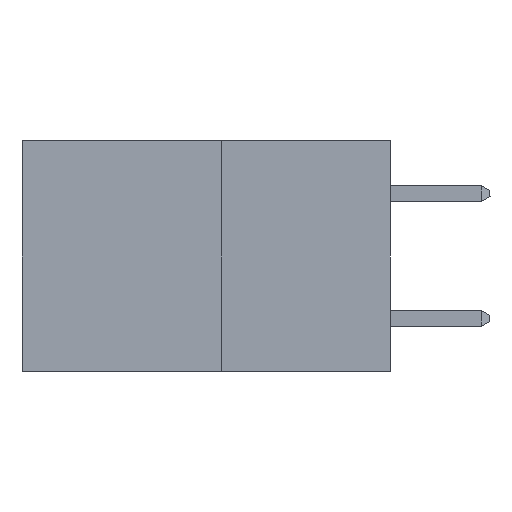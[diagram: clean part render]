
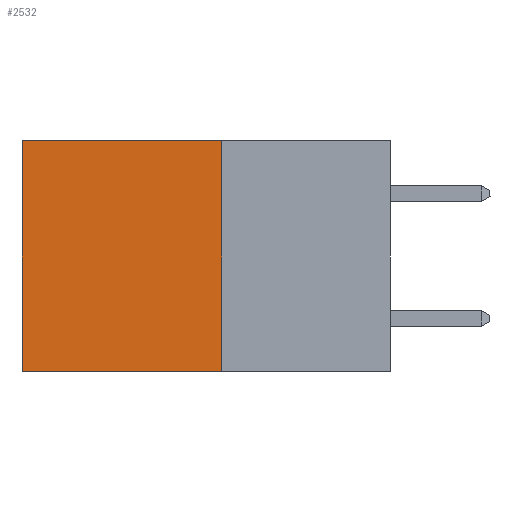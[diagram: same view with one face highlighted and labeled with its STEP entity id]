
A CAD part, left-side view. The second image highlights one B-rep face of the part: STEP entity #2532.
In plain terms, the highlighted planar face has unit normal (-1, 0, 0).
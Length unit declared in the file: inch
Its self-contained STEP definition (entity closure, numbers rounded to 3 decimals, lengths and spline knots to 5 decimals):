
#1038 = LINE ( 'NONE', #13134, #4888 ) ;
#1607 = LINE ( 'NONE', #19316, #9572 ) ;
#2513 = EDGE_CURVE ( 'NONE', #14275, #5086, #7500, .T. ) ;
#2532 = ADVANCED_FACE ( 'NONE', ( #10692 ), #6028, .F. ) ;
#2964 = VERTEX_POINT ( 'NONE', #14074 ) ;
#3160 = ORIENTED_EDGE ( 'NONE', *, *, #2513, .F. ) ;
#3594 = EDGE_LOOP ( 'NONE', ( #10285, #3160, #4442, #5634 ) ) ;
#3852 = VERTEX_POINT ( 'NONE', #9405 ) ;
#4442 = ORIENTED_EDGE ( 'NONE', *, *, #13285, .F. ) ;
#4865 = CARTESIAN_POINT ( 'NONE',  ( 0.277, 0.27, -0.37 ) ) ;
#4888 = VECTOR ( 'NONE', #13001, 39.37008 ) ;
#5086 = VERTEX_POINT ( 'NONE', #18165 ) ;
#5318 = LINE ( 'NONE', #10548, #17560 ) ;
#5634 = ORIENTED_EDGE ( 'NONE', *, *, #14609, .T. ) ;
#6028 = PLANE ( 'NONE',  #13375 ) ;
#6698 = CARTESIAN_POINT ( 'NONE',  ( 0.277, 0.27, -0.37 ) ) ;
#7036 = DIRECTION ( 'NONE',  ( 0., 1., 0. ) ) ;
#7055 = DIRECTION ( 'NONE',  ( 1., 0., 0. ) ) ;
#7500 = LINE ( 'NONE', #4865, #16031 ) ;
#9405 = CARTESIAN_POINT ( 'NONE',  ( 0.277, 0.27, 0. ) ) ;
#9572 = VECTOR ( 'NONE', #19127, 39.37008 ) ;
#10285 = ORIENTED_EDGE ( 'NONE', *, *, #15844, .T. ) ;
#10548 = CARTESIAN_POINT ( 'NONE',  ( 0.277, 0.59, -0.37 ) ) ;
#10692 = FACE_OUTER_BOUND ( 'NONE', #3594, .T. ) ;
#13001 = DIRECTION ( 'NONE',  ( 0., 1., 0. ) ) ;
#13065 = DIRECTION ( 'NONE',  ( 0., 0., -1. ) ) ;
#13134 = CARTESIAN_POINT ( 'NONE',  ( 0.277, 0.27, 0. ) ) ;
#13285 = EDGE_CURVE ( 'NONE', #3852, #14275, #1607, .T. ) ;
#13375 = AXIS2_PLACEMENT_3D ( 'NONE', #6698, #7055, #13065 ) ;
#14074 = CARTESIAN_POINT ( 'NONE',  ( 0.277, 0.59, 0. ) ) ;
#14275 = VERTEX_POINT ( 'NONE', #17128 ) ;
#14609 = EDGE_CURVE ( 'NONE', #3852, #2964, #1038, .T. ) ;
#15388 = DIRECTION ( 'NONE',  ( 0., 0., -1. ) ) ;
#15844 = EDGE_CURVE ( 'NONE', #2964, #5086, #5318, .T. ) ;
#16031 = VECTOR ( 'NONE', #7036, 39.37008 ) ;
#17128 = CARTESIAN_POINT ( 'NONE',  ( 0.277, 0.27, -0.37 ) ) ;
#17560 = VECTOR ( 'NONE', #15388, 39.37008 ) ;
#18165 = CARTESIAN_POINT ( 'NONE',  ( 0.277, 0.59, -0.37 ) ) ;
#19127 = DIRECTION ( 'NONE',  ( 0., 0., -1. ) ) ;
#19316 = CARTESIAN_POINT ( 'NONE',  ( 0.277, 0.27, -0.37 ) ) ;
